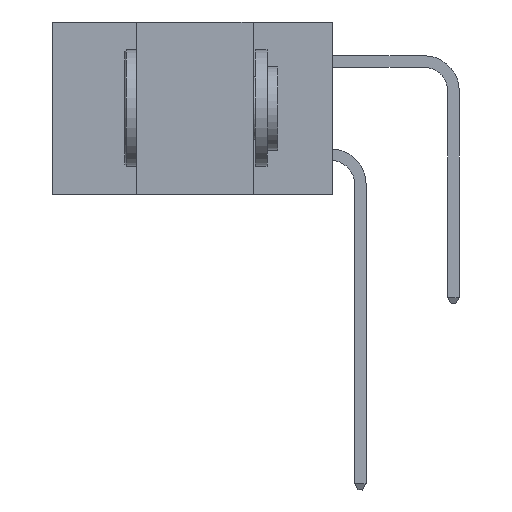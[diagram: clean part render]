
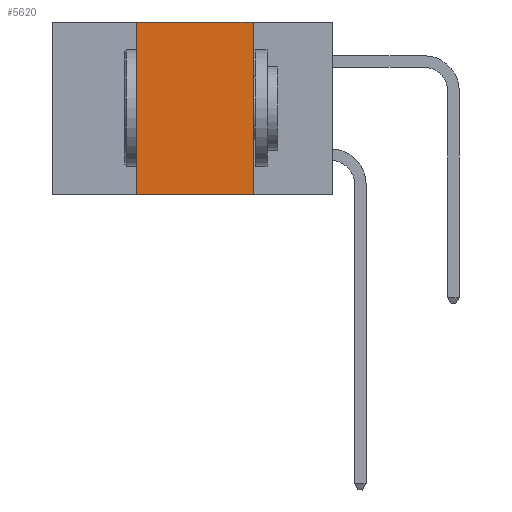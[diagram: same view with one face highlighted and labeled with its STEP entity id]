
A CAD part, left-side view. The second image highlights one B-rep face of the part: STEP entity #5620.
In plain terms, the highlighted planar face has unit normal (-1, 0, 0).
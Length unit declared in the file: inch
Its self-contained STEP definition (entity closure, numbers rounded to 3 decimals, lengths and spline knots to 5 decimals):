
#2118 = ORIENTED_EDGE ( 'NONE', *, *, #17384, .F. ) ;
#3051 = EDGE_CURVE ( 'NONE', #15560, #4624, #22777, .T. ) ;
#3055 = CARTESIAN_POINT ( 'NONE',  ( 0., 0.6, 0. ) ) ;
#3228 = LINE ( 'NONE', #7532, #5226 ) ;
#3788 = ORIENTED_EDGE ( 'NONE', *, *, #10462, .T. ) ;
#4042 = LINE ( 'NONE', #4434, #12531 ) ;
#4434 = CARTESIAN_POINT ( 'NONE',  ( 0., 0.6, -0.37 ) ) ;
#4484 = EDGE_LOOP ( 'NONE', ( #9292, #2118, #18009, #3788 ) ) ;
#4624 = VERTEX_POINT ( 'NONE', #22226 ) ;
#5226 = VECTOR ( 'NONE', #24061, 39.37008 ) ;
#5602 = DIRECTION ( 'NONE',  ( 1., 0., 0. ) ) ;
#5620 = ADVANCED_FACE ( 'NONE', ( #7642 ), #24038, .F. ) ;
#7532 = CARTESIAN_POINT ( 'NONE',  ( 0., 0.42, -0.37 ) ) ;
#7611 = VERTEX_POINT ( 'NONE', #18904 ) ;
#7642 = FACE_OUTER_BOUND ( 'NONE', #4484, .T. ) ;
#8402 = CARTESIAN_POINT ( 'NONE',  ( 0., 0.6, 0. ) ) ;
#8417 = VECTOR ( 'NONE', #8531, 39.37008 ) ;
#8531 = DIRECTION ( 'NONE',  ( 0., -1., 0. ) ) ;
#9292 = ORIENTED_EDGE ( 'NONE', *, *, #3051, .F. ) ;
#10462 = EDGE_CURVE ( 'NONE', #13011, #4624, #4042, .T. ) ;
#10625 = DIRECTION ( 'NONE',  ( 0., -1., 0. ) ) ;
#12302 = CARTESIAN_POINT ( 'NONE',  ( 0., 0.17, -0.37 ) ) ;
#12531 = VECTOR ( 'NONE', #10625, 39.37008 ) ;
#12560 = DIRECTION ( 'NONE',  ( 0., 0., -1. ) ) ;
#12850 = EDGE_CURVE ( 'NONE', #13011, #7611, #3228, .T. ) ;
#13011 = VERTEX_POINT ( 'NONE', #16533 ) ;
#15560 = VERTEX_POINT ( 'NONE', #25066 ) ;
#16533 = CARTESIAN_POINT ( 'NONE',  ( 0., 0.42, -0.37 ) ) ;
#17384 = EDGE_CURVE ( 'NONE', #7611, #15560, #24916, .T. ) ;
#18009 = ORIENTED_EDGE ( 'NONE', *, *, #12850, .F. ) ;
#18904 = CARTESIAN_POINT ( 'NONE',  ( 0., 0.42, 0. ) ) ;
#19240 = AXIS2_PLACEMENT_3D ( 'NONE', #3055, #5602, #22032 ) ;
#22032 = DIRECTION ( 'NONE',  ( 0., 0., -1. ) ) ;
#22226 = CARTESIAN_POINT ( 'NONE',  ( 0., 0.17, -0.37 ) ) ;
#22486 = VECTOR ( 'NONE', #12560, 39.37008 ) ;
#22777 = LINE ( 'NONE', #12302, #22486 ) ;
#24038 = PLANE ( 'NONE',  #19240 ) ;
#24061 = DIRECTION ( 'NONE',  ( 0., 0., 1. ) ) ;
#24916 = LINE ( 'NONE', #8402, #8417 ) ;
#25066 = CARTESIAN_POINT ( 'NONE',  ( 0., 0.17, 0. ) ) ;
